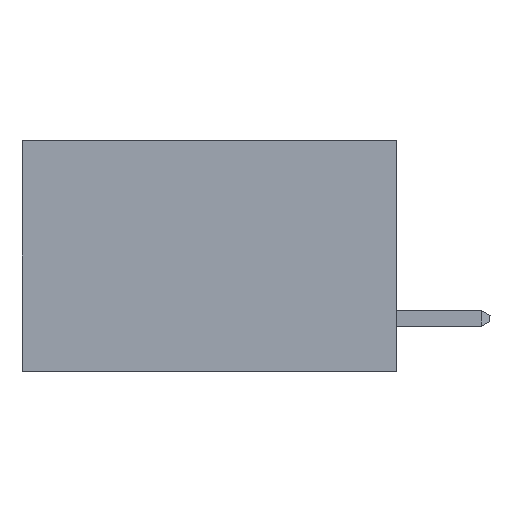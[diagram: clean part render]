
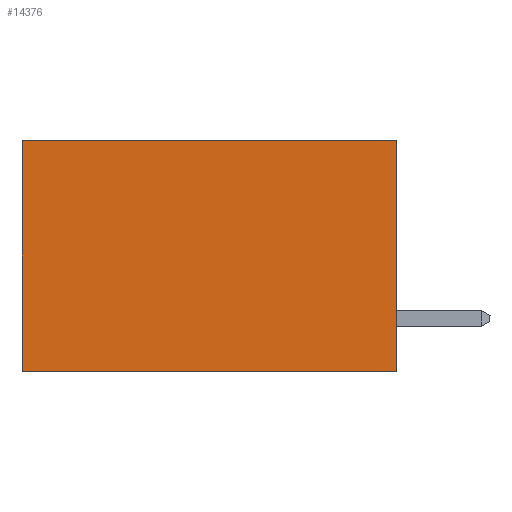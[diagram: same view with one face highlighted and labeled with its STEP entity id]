
A CAD part, left-side view. The second image highlights one B-rep face of the part: STEP entity #14376.
In plain terms, the highlighted planar face has unit normal (-1, 0, 0).
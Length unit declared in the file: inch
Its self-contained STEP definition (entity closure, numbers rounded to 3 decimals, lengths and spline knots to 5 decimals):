
#791 = VERTEX_POINT ( 'NONE', #2040 ) ;
#1177 = DIRECTION ( 'NONE',  ( 0., 0., -1. ) ) ;
#1842 = EDGE_CURVE ( 'NONE', #21843, #16354, #23375, .T. ) ;
#1872 = CARTESIAN_POINT ( 'NONE',  ( 0.298, 0., 0. ) ) ;
#2040 = CARTESIAN_POINT ( 'NONE',  ( 0.298, 0.6, 0. ) ) ;
#2226 = ORIENTED_EDGE ( 'NONE', *, *, #4518, .T. ) ;
#2508 = DIRECTION ( 'NONE',  ( 0., 0., -1. ) ) ;
#3133 = FACE_OUTER_BOUND ( 'NONE', #17168, .T. ) ;
#4365 = EDGE_CURVE ( 'NONE', #20352, #21843, #22547, .T. ) ;
#4431 = VECTOR ( 'NONE', #22595, 39.37008 ) ;
#4518 = EDGE_CURVE ( 'NONE', #791, #16354, #13702, .T. ) ;
#6517 = ORIENTED_EDGE ( 'NONE', *, *, #4365, .F. ) ;
#7208 = CARTESIAN_POINT ( 'NONE',  ( 0.298, 0.6, 0. ) ) ;
#9706 = LINE ( 'NONE', #24788, #4431 ) ;
#10503 = DIRECTION ( 'NONE',  ( 1., 0., 0. ) ) ;
#12478 = PLANE ( 'NONE',  #25179 ) ;
#12516 = CARTESIAN_POINT ( 'NONE',  ( 0.298, 0., -0.37 ) ) ;
#12528 = CARTESIAN_POINT ( 'NONE',  ( 0.298, 0.6, -0.37 ) ) ;
#13702 = LINE ( 'NONE', #7208, #23497 ) ;
#14376 = ADVANCED_FACE ( 'NONE', ( #3133 ), #12478, .F. ) ;
#14389 = DIRECTION ( 'NONE',  ( 0., 1., 0. ) ) ;
#14925 = VECTOR ( 'NONE', #15657, 39.37008 ) ;
#15576 = CARTESIAN_POINT ( 'NONE',  ( 0.298, 0., 0. ) ) ;
#15657 = DIRECTION ( 'NONE',  ( 0., 0., -1. ) ) ;
#16166 = CARTESIAN_POINT ( 'NONE',  ( 0.298, 0., 0. ) ) ;
#16354 = VERTEX_POINT ( 'NONE', #12528 ) ;
#17168 = EDGE_LOOP ( 'NONE', ( #2226, #17523, #6517, #23764 ) ) ;
#17361 = EDGE_CURVE ( 'NONE', #20352, #791, #9706, .T. ) ;
#17523 = ORIENTED_EDGE ( 'NONE', *, *, #1842, .F. ) ;
#20352 = VERTEX_POINT ( 'NONE', #1872 ) ;
#21250 = VECTOR ( 'NONE', #14389, 39.37008 ) ;
#21843 = VERTEX_POINT ( 'NONE', #22193 ) ;
#22193 = CARTESIAN_POINT ( 'NONE',  ( 0.298, 0., -0.37 ) ) ;
#22547 = LINE ( 'NONE', #15576, #14925 ) ;
#22595 = DIRECTION ( 'NONE',  ( 0., 1., 0. ) ) ;
#23375 = LINE ( 'NONE', #12516, #21250 ) ;
#23497 = VECTOR ( 'NONE', #1177, 39.37008 ) ;
#23764 = ORIENTED_EDGE ( 'NONE', *, *, #17361, .T. ) ;
#24788 = CARTESIAN_POINT ( 'NONE',  ( 0.298, 0., 0. ) ) ;
#25179 = AXIS2_PLACEMENT_3D ( 'NONE', #16166, #10503, #2508 ) ;
